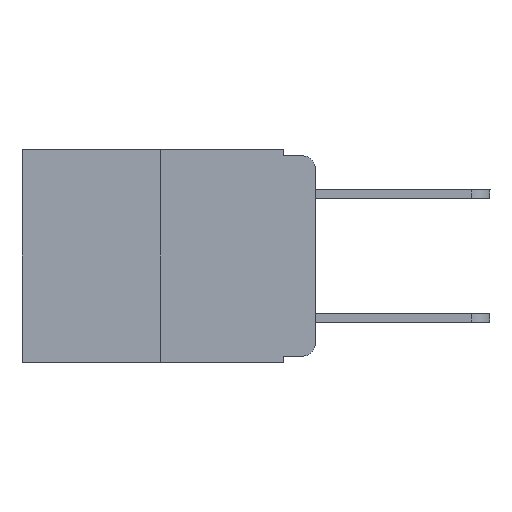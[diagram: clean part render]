
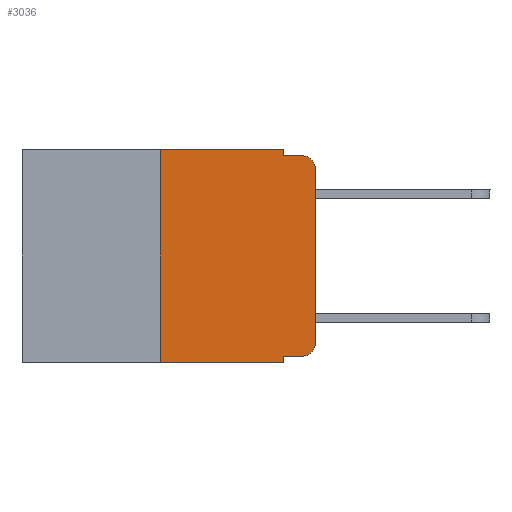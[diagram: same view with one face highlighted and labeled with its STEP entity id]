
A CAD part, left-side view. The second image highlights one B-rep face of the part: STEP entity #3036.
In plain terms, the highlighted planar face has unit normal (-1, 0, 0).
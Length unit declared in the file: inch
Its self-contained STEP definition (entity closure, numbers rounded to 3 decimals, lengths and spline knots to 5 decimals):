
#733 = FACE_OUTER_BOUND ( 'NONE', #4175, .T. ) ;
#757 = CARTESIAN_POINT ( 'NONE',  ( 0., 0., -0.313 ) ) ;
#806 = VERTEX_POINT ( 'NONE', #6004 ) ;
#881 = DIRECTION ( 'NONE',  ( 0., -1., 0. ) ) ;
#1266 = EDGE_CURVE ( 'NONE', #11505, #6470, #15840, .T. ) ;
#1419 = EDGE_CURVE ( 'NONE', #6470, #13562, #15103, .T. ) ;
#1764 = ORIENTED_EDGE ( 'NONE', *, *, #12892, .F. ) ;
#1808 = EDGE_CURVE ( 'NONE', #806, #10231, #2250, .T. ) ;
#2075 = DIRECTION ( 'NONE',  ( 0., 0., -1. ) ) ;
#2143 = EDGE_CURVE ( 'NONE', #7121, #10720, #6025, .T. ) ;
#2250 = LINE ( 'NONE', #9034, #14976 ) ;
#2261 = CARTESIAN_POINT ( 'NONE',  ( 0., 0.051, -0.343 ) ) ;
#2274 = ORIENTED_EDGE ( 'NONE', *, *, #7741, .T. ) ;
#2671 = LINE ( 'NONE', #9534, #10691 ) ;
#3036 = ADVANCED_FACE ( 'NONE', ( #733 ), #4952, .F. ) ;
#3048 = DIRECTION ( 'NONE',  ( 0., 0., -1. ) ) ;
#3167 = VECTOR ( 'NONE', #17412, 39.37008 ) ;
#3280 = DIRECTION ( 'NONE',  ( 0., 0., 1. ) ) ;
#3320 = DIRECTION ( 'NONE',  ( -1., 0., 0. ) ) ;
#3406 = CARTESIAN_POINT ( 'NONE',  ( 0., 0.02, -0.333 ) ) ;
#3484 = EDGE_CURVE ( 'NONE', #10231, #10619, #11994, .T. ) ;
#3828 = CARTESIAN_POINT ( 'NONE',  ( 0., 0.051, -0.01 ) ) ;
#3834 = VERTEX_POINT ( 'NONE', #11449 ) ;
#4175 = EDGE_LOOP ( 'NONE', ( #13041, #2274, #10311, #10837, #1764, #16154, #17253, #9906, #5224, #15040 ) ) ;
#4231 = VERTEX_POINT ( 'NONE', #11234 ) ;
#4952 = PLANE ( 'NONE',  #17051 ) ;
#4996 = AXIS2_PLACEMENT_3D ( 'NONE', #11629, #3320, #3048 ) ;
#5038 = DIRECTION ( 'NONE',  ( 1., 0., 0. ) ) ;
#5158 = VECTOR ( 'NONE', #13958, 39.37008 ) ;
#5224 = ORIENTED_EDGE ( 'NONE', *, *, #14631, .T. ) ;
#6004 = CARTESIAN_POINT ( 'NONE',  ( 0., 0.051, 0. ) ) ;
#6025 = LINE ( 'NONE', #10284, #3167 ) ;
#6274 = EDGE_CURVE ( 'NONE', #4231, #10720, #7722, .T. ) ;
#6470 = VERTEX_POINT ( 'NONE', #757 ) ;
#7028 = CARTESIAN_POINT ( 'NONE',  ( 0., 0.25, -0.343 ) ) ;
#7121 = VERTEX_POINT ( 'NONE', #7028 ) ;
#7722 = LINE ( 'NONE', #15802, #8439 ) ;
#7741 = EDGE_CURVE ( 'NONE', #13562, #10619, #10227, .T. ) ;
#8333 = VECTOR ( 'NONE', #9677, 39.37008 ) ;
#8439 = VECTOR ( 'NONE', #13233, 39.37008 ) ;
#9000 = VECTOR ( 'NONE', #3280, 39.37008 ) ;
#9034 = CARTESIAN_POINT ( 'NONE',  ( 0., 0.051, 0. ) ) ;
#9413 = CARTESIAN_POINT ( 'NONE',  ( 0., 0., 0. ) ) ;
#9534 = CARTESIAN_POINT ( 'NONE',  ( 0., 0.051, -0.333 ) ) ;
#9555 = CARTESIAN_POINT ( 'NONE',  ( 0., 0.473, 0. ) ) ;
#9677 = DIRECTION ( 'NONE',  ( 0., 0., 1. ) ) ;
#9906 = ORIENTED_EDGE ( 'NONE', *, *, #6274, .F. ) ;
#10227 = CIRCLE ( 'NONE', #4996, 0.02 ) ;
#10231 = VERTEX_POINT ( 'NONE', #3828 ) ;
#10284 = CARTESIAN_POINT ( 'NONE',  ( 0., 0.473, -0.343 ) ) ;
#10285 = CARTESIAN_POINT ( 'NONE',  ( 0., 0.051, -0.01 ) ) ;
#10311 = ORIENTED_EDGE ( 'NONE', *, *, #3484, .F. ) ;
#10405 = CARTESIAN_POINT ( 'NONE',  ( 0., 0.02, -0.01 ) ) ;
#10481 = DIRECTION ( 'NONE',  ( 0., 0., -1. ) ) ;
#10499 = CARTESIAN_POINT ( 'NONE',  ( 0., 0.02, -0.313 ) ) ;
#10619 = VERTEX_POINT ( 'NONE', #10405 ) ;
#10691 = VECTOR ( 'NONE', #16221, 39.37008 ) ;
#10720 = VERTEX_POINT ( 'NONE', #2261 ) ;
#10837 = ORIENTED_EDGE ( 'NONE', *, *, #1808, .F. ) ;
#11234 = CARTESIAN_POINT ( 'NONE',  ( 0., 0.051, -0.333 ) ) ;
#11449 = CARTESIAN_POINT ( 'NONE',  ( 0., 0.25, 0. ) ) ;
#11505 = VERTEX_POINT ( 'NONE', #3406 ) ;
#11629 = CARTESIAN_POINT ( 'NONE',  ( 0., 0.02, -0.03 ) ) ;
#11682 = DIRECTION ( 'NONE',  ( 0., 0., -1. ) ) ;
#11760 = CARTESIAN_POINT ( 'NONE',  ( 0., 0.25, 0. ) ) ;
#11994 = LINE ( 'NONE', #10285, #14452 ) ;
#12422 = CARTESIAN_POINT ( 'NONE',  ( 0., 0., -0.03 ) ) ;
#12892 = EDGE_CURVE ( 'NONE', #3834, #806, #17689, .T. ) ;
#13041 = ORIENTED_EDGE ( 'NONE', *, *, #1419, .T. ) ;
#13187 = LINE ( 'NONE', #11760, #9000 ) ;
#13233 = DIRECTION ( 'NONE',  ( 0., 0., -1. ) ) ;
#13562 = VERTEX_POINT ( 'NONE', #12422 ) ;
#13958 = DIRECTION ( 'NONE',  ( 0., -1., 0. ) ) ;
#14452 = VECTOR ( 'NONE', #881, 39.37008 ) ;
#14631 = EDGE_CURVE ( 'NONE', #4231, #11505, #2671, .T. ) ;
#14976 = VECTOR ( 'NONE', #2075, 39.37008 ) ;
#15040 = ORIENTED_EDGE ( 'NONE', *, *, #1266, .T. ) ;
#15103 = LINE ( 'NONE', #9413, #8333 ) ;
#15802 = CARTESIAN_POINT ( 'NONE',  ( 0., 0.051, 0. ) ) ;
#15840 = CIRCLE ( 'NONE', #17273, 0.02 ) ;
#16154 = ORIENTED_EDGE ( 'NONE', *, *, #16804, .F. ) ;
#16221 = DIRECTION ( 'NONE',  ( 0., -1., 0. ) ) ;
#16804 = EDGE_CURVE ( 'NONE', #7121, #3834, #13187, .T. ) ;
#17051 = AXIS2_PLACEMENT_3D ( 'NONE', #17175, #5038, #10481 ) ;
#17175 = CARTESIAN_POINT ( 'NONE',  ( 0., 0.473, 0. ) ) ;
#17253 = ORIENTED_EDGE ( 'NONE', *, *, #2143, .T. ) ;
#17273 = AXIS2_PLACEMENT_3D ( 'NONE', #10499, #17460, #11682 ) ;
#17412 = DIRECTION ( 'NONE',  ( 0., -1., 0. ) ) ;
#17460 = DIRECTION ( 'NONE',  ( -1., 0., 0. ) ) ;
#17689 = LINE ( 'NONE', #9555, #5158 ) ;
